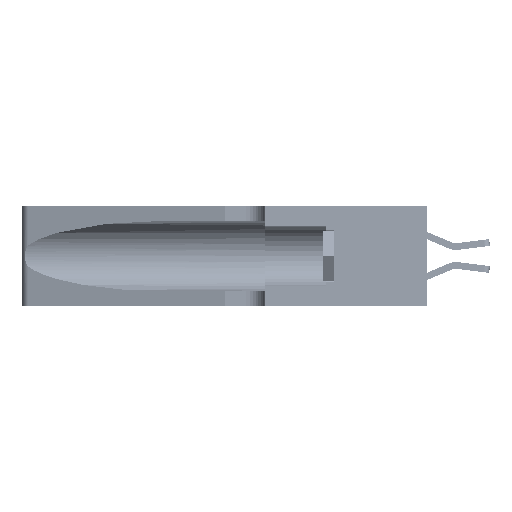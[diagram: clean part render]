
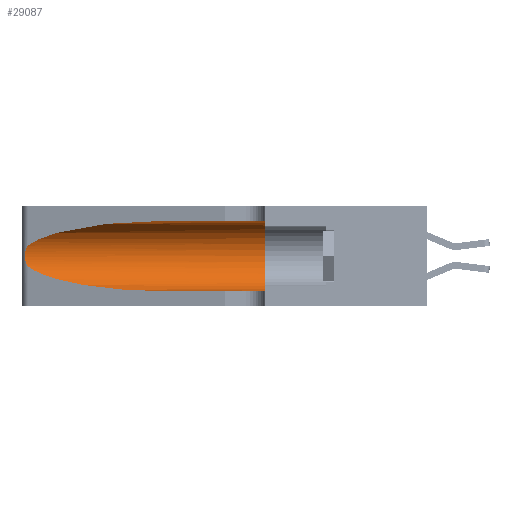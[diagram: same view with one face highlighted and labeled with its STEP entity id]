
A CAD part, left-side view. The second image highlights one B-rep face of the part: STEP entity #29087.
In plain terms, the highlighted cylindrical face has radius 3.308 mm (diameter 6.617 mm), a partial arc.
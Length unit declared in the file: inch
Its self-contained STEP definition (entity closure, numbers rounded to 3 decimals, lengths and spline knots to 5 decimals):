
#37 = CARTESIAN_POINT ( 'NONE',  ( 0.25639, 1.23186, 0.15144 ) ) ;
#589 = CARTESIAN_POINT ( 'NONE',  ( 0.1305, 0.35, 0.31525 ) ) ;
#1134 = CARTESIAN_POINT ( 'NONE',  ( 0.25487, 1.22718, 0.14631 ) ) ;
#1229 = DIRECTION ( 'NONE',  ( 0., 0., 1. ) ) ;
#1385 = EDGE_LOOP ( 'NONE', ( #6698, #36288, #5478, #34816, #20711, #23312 ) ) ;
#1632 = LINE ( 'NONE', #4851, #38577 ) ;
#1635 = EDGE_CURVE ( 'NONE', #37881, #7990, #18798, .T. ) ;
#3108 = CARTESIAN_POINT ( 'NONE',  ( 0.1305, 0.72297, 0.05475 ) ) ;
#3497 = VECTOR ( 'NONE', #35013, 39.37008 ) ;
#4851 = CARTESIAN_POINT ( 'NONE',  ( 0.1305, 1.61858, 0.31525 ) ) ;
#5436 = CARTESIAN_POINT ( 'NONE',  ( 0.25487, 1.22718, 0.14631 ) ) ;
#5478 = ORIENTED_EDGE ( 'NONE', *, *, #11087, .T. ) ;
#6172 = CYLINDRICAL_SURFACE ( 'NONE', #23899, 0.13025 ) ;
#6698 = ORIENTED_EDGE ( 'NONE', *, *, #16105, .T. ) ;
#7121 = FACE_OUTER_BOUND ( 'NONE', #1385, .T. ) ;
#7426 = CARTESIAN_POINT ( 'NONE',  ( 0.26017, 1.23833, 0.17102 ) ) ;
#7827 = CARTESIAN_POINT ( 'NONE',  ( 0.25487, 1.22718, 0.22369 ) ) ;
#7990 = VERTEX_POINT ( 'NONE', #5436 ) ;
#8564 = CARTESIAN_POINT ( 'NONE',  ( 0.2373, 1.15595, 0.28018 ) ) ;
#10758 = EDGE_CURVE ( 'NONE', #38716, #26132, #1632, .T. ) ;
#11087 = EDGE_CURVE ( 'NONE', #7990, #13549, #33849, .T. ) ;
#13549 = VERTEX_POINT ( 'NONE', #3108 ) ;
#13899 = CARTESIAN_POINT ( 'NONE',  ( 0.1305, 0.72297, 0.31525 ) ) ;
#14744 = CARTESIAN_POINT ( 'NONE',  ( 0.2373, 1.15595, 0.08982 ) ) ;
#14872 = CARTESIAN_POINT ( 'NONE',  ( 0.1305, 0.72297, 0.05475 ) ) ;
#15320 = CARTESIAN_POINT ( 'NONE',  ( 0.1305, 0.35, 0.05475 ) ) ;
#16105 = EDGE_CURVE ( 'NONE', #38716, #37881, #21396, .T. ) ;
#16327 = CARTESIAN_POINT ( 'NONE',  ( 0.26075, 1.23896, 0.178 ) ) ;
#16710 = CARTESIAN_POINT ( 'NONE',  ( 0.25639, 1.23184, 0.21858 ) ) ;
#17640 = CARTESIAN_POINT ( 'NONE',  ( 0.25487, 1.22718, 0.14631 ) ) ;
#18798 = B_SPLINE_CURVE_WITH_KNOTS ( 'NONE', 3,
 ( #7827, #34071, #16710, #22707, #28171, #31177, #34208, #16327, #7426, #28300, #31316, #37, #32901, #1134 ),
 .UNSPECIFIED., .F., .F.,
 ( 4, 2, 2, 2, 2, 2, 4 ),
 ( 0., 0.00027, 0.00053, 0.00107, 0.0016, 0.00187, 0.00214 ),
 .UNSPECIFIED. ) ;
#19001 = CARTESIAN_POINT ( 'NONE',  ( 0.1305, 0.72297, 0.31525 ) ) ;
#19603 = DIRECTION ( 'NONE',  ( 0., -1., 0. ) ) ;
#20711 = ORIENTED_EDGE ( 'NONE', *, *, #32477, .F. ) ;
#21396 =( BOUNDED_CURVE ( )  B_SPLINE_CURVE ( 3, ( #13899, #35345, #8564, #34828 ),
 .UNSPECIFIED., .F., .F. ) 
 B_SPLINE_CURVE_WITH_KNOTS ( ( 4, 4 ),
 ( 1.5708, 2.84003 ),
 .UNSPECIFIED. ) 
 CURVE ( )  GEOMETRIC_REPRESENTATION_ITEM ( )  RATIONAL_B_SPLINE_CURVE ( ( 1., 0.87, 0.87, 1. ) ) 
 REPRESENTATION_ITEM ( '' )  );
#21673 = CARTESIAN_POINT ( 'NONE',  ( 0.1305, 0.35, 0.185 ) ) ;
#22210 = LINE ( 'NONE', #34887, #3497 ) ;
#22707 = CARTESIAN_POINT ( 'NONE',  ( 0.25787, 1.23484, 0.2124 ) ) ;
#23312 = ORIENTED_EDGE ( 'NONE', *, *, #10758, .F. ) ;
#23899 = AXIS2_PLACEMENT_3D ( 'NONE', #28222, #19603, #26714 ) ;
#25680 = VERTEX_POINT ( 'NONE', #15320 ) ;
#26132 = VERTEX_POINT ( 'NONE', #589 ) ;
#26714 = DIRECTION ( 'NONE',  ( 0., 0., -1. ) ) ;
#28171 = CARTESIAN_POINT ( 'NONE',  ( 0.25854, 1.2359, 0.20912 ) ) ;
#28222 = CARTESIAN_POINT ( 'NONE',  ( 0.1305, 1.61858, 0.185 ) ) ;
#28300 = CARTESIAN_POINT ( 'NONE',  ( 0.25856, 1.23593, 0.16098 ) ) ;
#29087 = ADVANCED_FACE ( 'NONE', ( #7121 ), #6172, .F. ) ;
#29184 = CARTESIAN_POINT ( 'NONE',  ( 0.25487, 1.22718, 0.22369 ) ) ;
#30512 = DIRECTION ( 'NONE',  ( 0., 1., 0. ) ) ;
#31177 = CARTESIAN_POINT ( 'NONE',  ( 0.26018, 1.23835, 0.19895 ) ) ;
#31316 = CARTESIAN_POINT ( 'NONE',  ( 0.25789, 1.23486, 0.15765 ) ) ;
#31719 = DIRECTION ( 'NONE',  ( 0., -1., 0. ) ) ;
#32477 = EDGE_CURVE ( 'NONE', #26132, #25680, #37989, .T. ) ;
#32756 = CARTESIAN_POINT ( 'NONE',  ( 0.18966, 0.96281, 0.05475 ) ) ;
#32901 = CARTESIAN_POINT ( 'NONE',  ( 0.25555, 1.22993, 0.14849 ) ) ;
#33849 =( BOUNDED_CURVE ( )  B_SPLINE_CURVE ( 3, ( #17640, #14744, #32756, #14872 ),
 .UNSPECIFIED., .F., .F. ) 
 B_SPLINE_CURVE_WITH_KNOTS ( ( 4, 4 ),
 ( 3.44316, 4.71239 ),
 .UNSPECIFIED. ) 
 CURVE ( )  GEOMETRIC_REPRESENTATION_ITEM ( )  RATIONAL_B_SPLINE_CURVE ( ( 1., 0.87, 0.87, 1. ) ) 
 REPRESENTATION_ITEM ( '' )  );
#34071 = CARTESIAN_POINT ( 'NONE',  ( 0.25555, 1.22994, 0.2215 ) ) ;
#34208 = CARTESIAN_POINT ( 'NONE',  ( 0.26075, 1.23896, 0.19203 ) ) ;
#34816 = ORIENTED_EDGE ( 'NONE', *, *, #37207, .T. ) ;
#34828 = CARTESIAN_POINT ( 'NONE',  ( 0.25487, 1.22718, 0.22369 ) ) ;
#34887 = CARTESIAN_POINT ( 'NONE',  ( 0.1305, 1.61858, 0.05475 ) ) ;
#35013 = DIRECTION ( 'NONE',  ( 0., -1., 0. ) ) ;
#35345 = CARTESIAN_POINT ( 'NONE',  ( 0.18966, 0.96281, 0.31525 ) ) ;
#35453 = AXIS2_PLACEMENT_3D ( 'NONE', #21673, #30512, #1229 ) ;
#36288 = ORIENTED_EDGE ( 'NONE', *, *, #1635, .T. ) ;
#37207 = EDGE_CURVE ( 'NONE', #13549, #25680, #22210, .T. ) ;
#37881 = VERTEX_POINT ( 'NONE', #29184 ) ;
#37989 = CIRCLE ( 'NONE', #35453, 0.13025 ) ;
#38577 = VECTOR ( 'NONE', #31719, 39.37008 ) ;
#38716 = VERTEX_POINT ( 'NONE', #19001 ) ;
